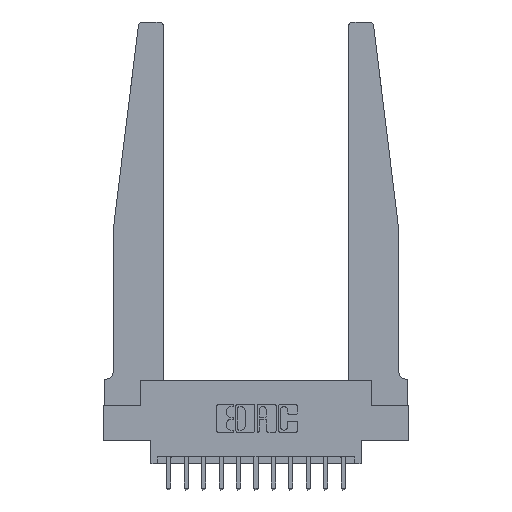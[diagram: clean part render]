
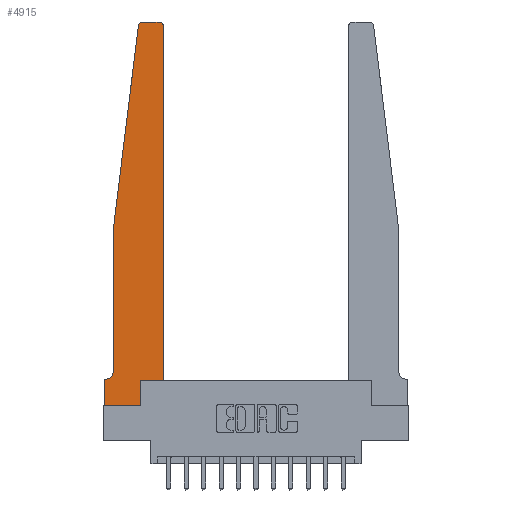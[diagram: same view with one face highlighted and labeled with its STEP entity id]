
A CAD part, top view. The second image highlights one B-rep face of the part: STEP entity #4915.
In plain terms, the highlighted planar face has unit normal (0, 0, 1).
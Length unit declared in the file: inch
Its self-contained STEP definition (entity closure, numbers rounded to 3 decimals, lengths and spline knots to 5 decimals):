
#249 = LINE ( 'NONE', #8591, #6496 ) ;
#298 = CARTESIAN_POINT ( 'NONE',  ( 0.27653, 2.72, 0.37 ) ) ;
#304 = CARTESIAN_POINT ( 'NONE',  ( 0.065, 0.1875, 0.37 ) ) ;
#358 = VECTOR ( 'NONE', #8373, 39.37008 ) ;
#362 = CARTESIAN_POINT ( 'NONE',  ( 0., 0.1875, 0.37 ) ) ;
#616 = AXIS2_PLACEMENT_3D ( 'NONE', #3386, #12277, #4637 ) ;
#660 = CARTESIAN_POINT ( 'NONE',  ( 0.065, 0.2375, 0.37 ) ) ;
#758 = LINE ( 'NONE', #4947, #13426 ) ;
#1137 = EDGE_CURVE ( 'NONE', #8272, #4392, #14218, .T. ) ;
#1164 = EDGE_CURVE ( 'NONE', #5536, #8272, #758, .T. ) ;
#1472 = VERTEX_POINT ( 'NONE', #15439 ) ;
#1575 = DIRECTION ( 'NONE',  ( 1., 0., 0. ) ) ;
#1847 = ORIENTED_EDGE ( 'NONE', *, *, #9228, .T. ) ;
#2036 = ORIENTED_EDGE ( 'NONE', *, *, #4746, .T. ) ;
#2145 = CARTESIAN_POINT ( 'NONE',  ( 0.2605, 0., 0.37 ) ) ;
#2277 = CARTESIAN_POINT ( 'NONE',  ( 0.015, 0.2375, 0.37 ) ) ;
#2573 = VECTOR ( 'NONE', #9085, 39.37008 ) ;
#3071 = EDGE_CURVE ( 'NONE', #1472, #11884, #3974, .T. ) ;
#3386 = CARTESIAN_POINT ( 'NONE',  ( 0., 0.1875, 0.37 ) ) ;
#3494 = DIRECTION ( 'NONE',  ( 0., 1., 0. ) ) ;
#3501 = DIRECTION ( 'NONE',  ( -1., 0., 0. ) ) ;
#3624 = CARTESIAN_POINT ( 'NONE',  ( 0.425, 0.18, 0.37 ) ) ;
#3676 = CARTESIAN_POINT ( 'NONE',  ( 0.065, 1.25, 0.37 ) ) ;
#3974 = LINE ( 'NONE', #3624, #13769 ) ;
#4069 = VERTEX_POINT ( 'NONE', #2145 ) ;
#4218 = AXIS2_PLACEMENT_3D ( 'NONE', #298, #9072, #1575 ) ;
#4229 = CARTESIAN_POINT ( 'NONE',  ( 0.25, 2.75, 0.37 ) ) ;
#4392 = VERTEX_POINT ( 'NONE', #660 ) ;
#4479 = VECTOR ( 'NONE', #6057, 39.37008 ) ;
#4637 = DIRECTION ( 'NONE',  ( 1., 0., 0. ) ) ;
#4697 = DIRECTION ( 'NONE',  ( -0.122, -0.992, 0. ) ) ;
#4746 = EDGE_CURVE ( 'NONE', #9903, #5536, #9700, .T. ) ;
#4877 = LINE ( 'NONE', #7297, #4479 ) ;
#4898 = DIRECTION ( 'NONE',  ( 0., -1., 0. ) ) ;
#4915 = ADVANCED_FACE ( 'NONE', ( #11887 ), #10990, .T. ) ;
#4947 = CARTESIAN_POINT ( 'NONE',  ( 0.065, 1.25, 0.37 ) ) ;
#5115 = CARTESIAN_POINT ( 'NONE',  ( 0.065, 1.25, 0.37 ) ) ;
#5382 = ORIENTED_EDGE ( 'NONE', *, *, #9530, .T. ) ;
#5536 = VERTEX_POINT ( 'NONE', #12534 ) ;
#5786 = AXIS2_PLACEMENT_3D ( 'NONE', #2277, #11103, #3501 ) ;
#6038 = EDGE_CURVE ( 'NONE', #10293, #4069, #4877, .T. ) ;
#6052 = DIRECTION ( 'NONE',  ( 0., -1., 0. ) ) ;
#6057 = DIRECTION ( 'NONE',  ( 1., 0., 0. ) ) ;
#6496 = VECTOR ( 'NONE', #9899, 39.37008 ) ;
#6725 = CARTESIAN_POINT ( 'NONE',  ( 0.425, 2.72, 0.37 ) ) ;
#6858 = LINE ( 'NONE', #4229, #12871 ) ;
#7001 = VECTOR ( 'NONE', #4898, 39.37008 ) ;
#7272 = ORIENTED_EDGE ( 'NONE', *, *, #1164, .T. ) ;
#7280 = VECTOR ( 'NONE', #6052, 39.37008 ) ;
#7297 = CARTESIAN_POINT ( 'NONE',  ( 0., 0., 0.37 ) ) ;
#7373 = VERTEX_POINT ( 'NONE', #12657 ) ;
#7382 = CARTESIAN_POINT ( 'NONE',  ( 0.395, 2.72, 0.37 ) ) ;
#8172 = EDGE_LOOP ( 'NONE', ( #1847, #2036, #7272, #11514, #8601, #5382, #12899, #15845, #13846, #8907, #8261, #9742 ) ) ;
#8191 = EDGE_CURVE ( 'NONE', #9586, #10293, #13707, .T. ) ;
#8220 = EDGE_CURVE ( 'NONE', #7373, #1472, #249, .T. ) ;
#8261 = ORIENTED_EDGE ( 'NONE', *, *, #3071, .T. ) ;
#8272 = VERTEX_POINT ( 'NONE', #3676 ) ;
#8373 = DIRECTION ( 'NONE',  ( 0., 1., 0. ) ) ;
#8591 = CARTESIAN_POINT ( 'NONE',  ( 0.425, 0.18, 0.37 ) ) ;
#8601 = ORIENTED_EDGE ( 'NONE', *, *, #11489, .T. ) ;
#8672 = DIRECTION ( 'NONE',  ( 1., 0., 0. ) ) ;
#8907 = ORIENTED_EDGE ( 'NONE', *, *, #8220, .T. ) ;
#9072 = DIRECTION ( 'NONE',  ( 0., 0., 1. ) ) ;
#9085 = DIRECTION ( 'NONE',  ( -1., 0., 0. ) ) ;
#9228 = EDGE_CURVE ( 'NONE', #15387, #9903, #6858, .T. ) ;
#9530 = EDGE_CURVE ( 'NONE', #13118, #9586, #15236, .T. ) ;
#9586 = VERTEX_POINT ( 'NONE', #362 ) ;
#9606 = CIRCLE ( 'NONE', #5786, 0.05 ) ;
#9700 = CIRCLE ( 'NONE', #4218, 0.03 ) ;
#9742 = ORIENTED_EDGE ( 'NONE', *, *, #12890, .T. ) ;
#9899 = DIRECTION ( 'NONE',  ( 1., 0., 0. ) ) ;
#9903 = VERTEX_POINT ( 'NONE', #12286 ) ;
#10293 = VERTEX_POINT ( 'NONE', #12145 ) ;
#10427 = CARTESIAN_POINT ( 'NONE',  ( 0.015, 0.1875, 0.37 ) ) ;
#10509 = AXIS2_PLACEMENT_3D ( 'NONE', #7382, #16316, #8672 ) ;
#10913 = EDGE_CURVE ( 'NONE', #4069, #7373, #14219, .T. ) ;
#10990 = PLANE ( 'NONE',  #616 ) ;
#11103 = DIRECTION ( 'NONE',  ( 0., 0., -1. ) ) ;
#11489 = EDGE_CURVE ( 'NONE', #4392, #13118, #9606, .T. ) ;
#11514 = ORIENTED_EDGE ( 'NONE', *, *, #1137, .T. ) ;
#11884 = VERTEX_POINT ( 'NONE', #6725 ) ;
#11887 = FACE_OUTER_BOUND ( 'NONE', #8172, .T. ) ;
#12145 = CARTESIAN_POINT ( 'NONE',  ( 0., 0., 0.37 ) ) ;
#12240 = CARTESIAN_POINT ( 'NONE',  ( 0., 0., 0.37 ) ) ;
#12277 = DIRECTION ( 'NONE',  ( 0., 0., 1. ) ) ;
#12286 = CARTESIAN_POINT ( 'NONE',  ( 0.27653, 2.75, 0.37 ) ) ;
#12534 = CARTESIAN_POINT ( 'NONE',  ( 0.24675, 2.72367, 0.37 ) ) ;
#12657 = CARTESIAN_POINT ( 'NONE',  ( 0.2605, 0.18, 0.37 ) ) ;
#12871 = VECTOR ( 'NONE', #13166, 39.37008 ) ;
#12890 = EDGE_CURVE ( 'NONE', #11884, #15387, #14770, .T. ) ;
#12899 = ORIENTED_EDGE ( 'NONE', *, *, #8191, .T. ) ;
#13118 = VERTEX_POINT ( 'NONE', #10427 ) ;
#13166 = DIRECTION ( 'NONE',  ( -1., 0., 0. ) ) ;
#13426 = VECTOR ( 'NONE', #4697, 39.37008 ) ;
#13707 = LINE ( 'NONE', #12240, #7280 ) ;
#13736 = CARTESIAN_POINT ( 'NONE',  ( 0.395, 2.75, 0.37 ) ) ;
#13769 = VECTOR ( 'NONE', #3494, 39.37008 ) ;
#13846 = ORIENTED_EDGE ( 'NONE', *, *, #10913, .T. ) ;
#14218 = LINE ( 'NONE', #5115, #7001 ) ;
#14219 = LINE ( 'NONE', #16071, #358 ) ;
#14770 = CIRCLE ( 'NONE', #10509, 0.03 ) ;
#15236 = LINE ( 'NONE', #304, #2573 ) ;
#15387 = VERTEX_POINT ( 'NONE', #13736 ) ;
#15439 = CARTESIAN_POINT ( 'NONE',  ( 0.425, 0.18, 0.37 ) ) ;
#15845 = ORIENTED_EDGE ( 'NONE', *, *, #6038, .T. ) ;
#16071 = CARTESIAN_POINT ( 'NONE',  ( 0.2605, 0.18, 0.37 ) ) ;
#16316 = DIRECTION ( 'NONE',  ( 0., 0., 1. ) ) ;
